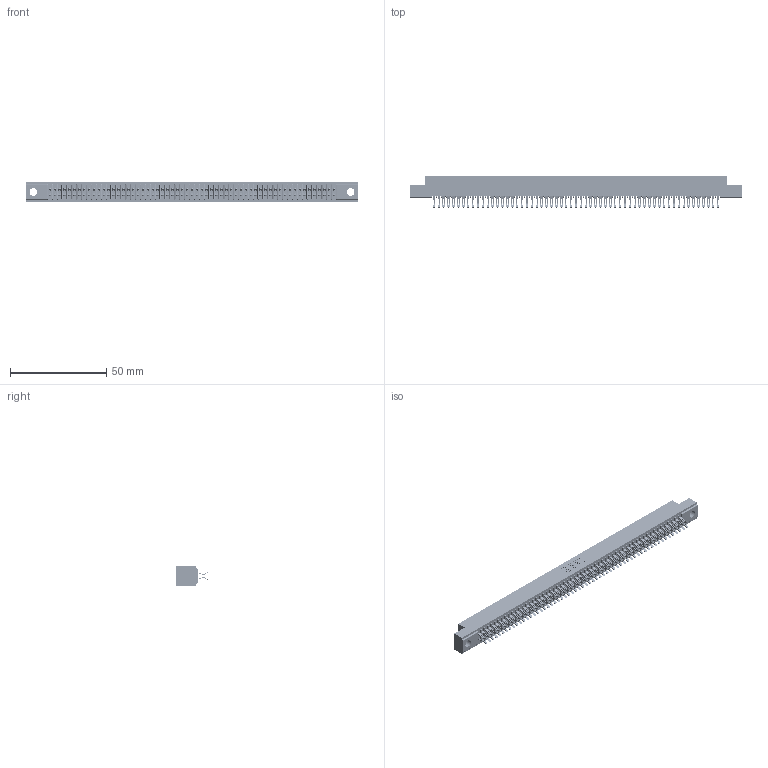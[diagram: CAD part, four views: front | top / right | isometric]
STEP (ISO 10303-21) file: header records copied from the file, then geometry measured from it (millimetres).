
FILE_DESCRIPTION (( 'STEP AP203' ), '1' );
FILE_NAME ('391-118-555-204.STEP', '2018-08-09T23:50:01', ( '' ), ( '' ), 'SwSTEP 2.0', 'SolidWorks 2016', '' );
FILE_SCHEMA (( 'CONFIG_CONTROL_DESIGN' ));
Length unit declared in the file: inch
Products named in the file (3): 341 Part_.156 (3.96) Dia Mounting Holes; 341-292-001_341-292-155; 391-118-555-204
Assembly tree (119 placements, depth 2):
  391-118-555-204
    341 Part_.156 (3.96) Dia Mounting Holes
    341-292-001_341-292-155  x118
Bounding box: 172.09 x 16.31 x 10.16 mm (x, y, z)
Volume: 12766.6 mm3; surface area: 24048.5 mm2
Topology: 119 solids, 119 shells, 9334 faces, 27905 edges, 18166 vertices
Faces by surface type: plane 5038, cylinder 4060, sphere 120, torus 116
Entity records: 70026 total; most frequent: CARTESIAN_POINT 11661, ORIENTED_EDGE 11578, DIRECTION 11287, EDGE_CURVE 5789, LINE 4687, VECTOR 4687, VERTEX_POINT 3658, AXIS2_PLACEMENT_3D 3300
